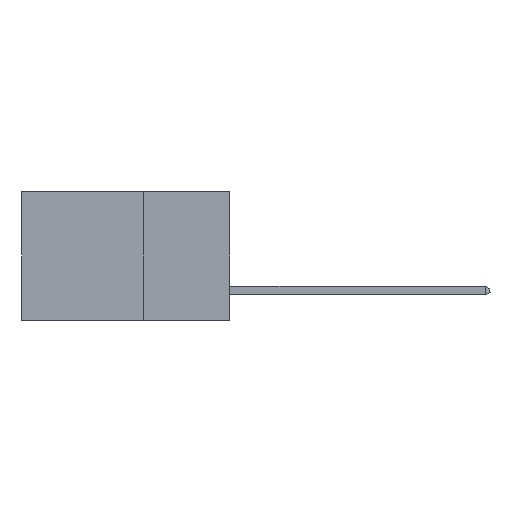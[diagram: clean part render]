
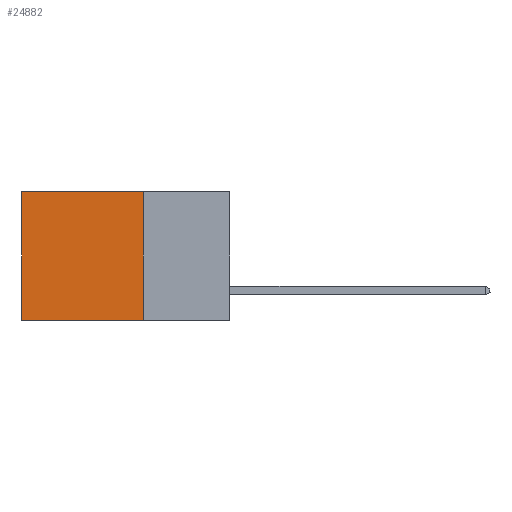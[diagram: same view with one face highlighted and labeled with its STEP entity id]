
A CAD part, left-side view. The second image highlights one B-rep face of the part: STEP entity #24882.
In plain terms, the highlighted planar face has unit normal (-1, 0, 0).
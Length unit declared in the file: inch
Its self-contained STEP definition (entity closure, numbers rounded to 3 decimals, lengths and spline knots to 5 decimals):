
#955 = AXIS2_PLACEMENT_3D ( 'NONE', #3543, #19498, #10731 ) ;
#1280 = DIRECTION ( 'NONE',  ( 0., 1., 0. ) ) ;
#3058 = LINE ( 'NONE', #21206, #25880 ) ;
#3543 = CARTESIAN_POINT ( 'NONE',  ( 0.298, 0.25, 0. ) ) ;
#3839 = DIRECTION ( 'NONE',  ( 0., 0., -1. ) ) ;
#4886 = EDGE_CURVE ( 'NONE', #15580, #8768, #18088, .T. ) ;
#5251 = EDGE_CURVE ( 'NONE', #23186, #15580, #25313, .T. ) ;
#6768 = CARTESIAN_POINT ( 'NONE',  ( 0.298, 0.25, 0. ) ) ;
#8195 = CARTESIAN_POINT ( 'NONE',  ( 0.298, 0.25, 0. ) ) ;
#8768 = VERTEX_POINT ( 'NONE', #19097 ) ;
#9322 = DIRECTION ( 'NONE',  ( 0., 0., -1. ) ) ;
#10224 = ORIENTED_EDGE ( 'NONE', *, *, #5251, .F. ) ;
#10731 = DIRECTION ( 'NONE',  ( 0., 0., -1. ) ) ;
#12657 = EDGE_CURVE ( 'NONE', #23186, #17632, #25405, .T. ) ;
#14991 = EDGE_LOOP ( 'NONE', ( #19731, #17773, #10224, #18688 ) ) ;
#15000 = VECTOR ( 'NONE', #1280, 39.37008 ) ;
#15026 = CARTESIAN_POINT ( 'NONE',  ( 0.298, 0.6, 0. ) ) ;
#15580 = VERTEX_POINT ( 'NONE', #27444 ) ;
#16306 = CARTESIAN_POINT ( 'NONE',  ( 0.298, 0.25, 0. ) ) ;
#17632 = VERTEX_POINT ( 'NONE', #15026 ) ;
#17727 = VECTOR ( 'NONE', #9322, 39.37008 ) ;
#17773 = ORIENTED_EDGE ( 'NONE', *, *, #4886, .F. ) ;
#18088 = LINE ( 'NONE', #23743, #15000 ) ;
#18688 = ORIENTED_EDGE ( 'NONE', *, *, #12657, .T. ) ;
#19097 = CARTESIAN_POINT ( 'NONE',  ( 0.298, 0.6, -0.37 ) ) ;
#19498 = DIRECTION ( 'NONE',  ( 1., 0., 0. ) ) ;
#19731 = ORIENTED_EDGE ( 'NONE', *, *, #23885, .T. ) ;
#20254 = FACE_OUTER_BOUND ( 'NONE', #14991, .T. ) ;
#21206 = CARTESIAN_POINT ( 'NONE',  ( 0.298, 0.6, 0. ) ) ;
#23186 = VERTEX_POINT ( 'NONE', #6768 ) ;
#23413 = DIRECTION ( 'NONE',  ( 0., 1., 0. ) ) ;
#23743 = CARTESIAN_POINT ( 'NONE',  ( 0.298, 0.25, -0.37 ) ) ;
#23885 = EDGE_CURVE ( 'NONE', #17632, #8768, #3058, .T. ) ;
#24675 = VECTOR ( 'NONE', #23413, 39.37008 ) ;
#24882 = ADVANCED_FACE ( 'NONE', ( #20254 ), #28597, .F. ) ;
#25313 = LINE ( 'NONE', #16306, #17727 ) ;
#25405 = LINE ( 'NONE', #8195, #24675 ) ;
#25880 = VECTOR ( 'NONE', #3839, 39.37008 ) ;
#27444 = CARTESIAN_POINT ( 'NONE',  ( 0.298, 0.25, -0.37 ) ) ;
#28597 = PLANE ( 'NONE',  #955 ) ;
